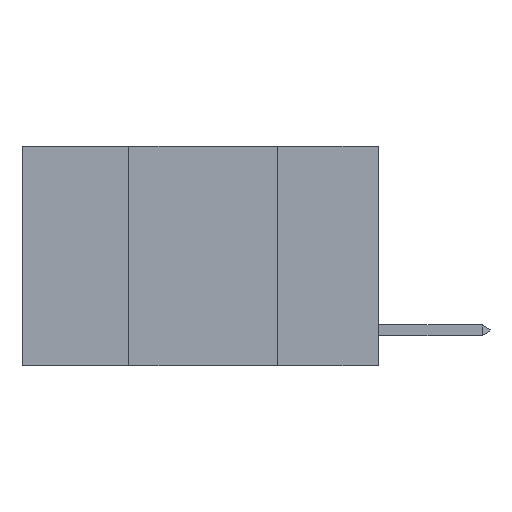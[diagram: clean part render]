
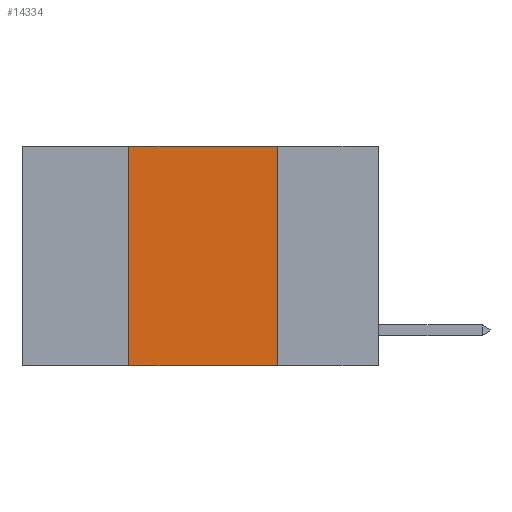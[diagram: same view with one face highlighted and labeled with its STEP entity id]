
A CAD part, left-side view. The second image highlights one B-rep face of the part: STEP entity #14334.
In plain terms, the highlighted planar face has unit normal (-1, 0, 0).
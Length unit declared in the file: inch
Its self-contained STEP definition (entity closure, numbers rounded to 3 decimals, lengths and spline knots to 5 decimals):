
#19 = DIRECTION ( 'NONE',  ( 0., 0., -1. ) ) ;
#130 = EDGE_LOOP ( 'NONE', ( #17119, #7793, #19392, #15109 ) ) ;
#524 = VECTOR ( 'NONE', #19965, 39.37008 ) ;
#1915 = VECTOR ( 'NONE', #15563, 39.37008 ) ;
#2830 = VERTEX_POINT ( 'NONE', #14378 ) ;
#3192 = DIRECTION ( 'NONE',  ( 0., -1., 0. ) ) ;
#3687 = PLANE ( 'NONE',  #16470 ) ;
#4139 = VERTEX_POINT ( 'NONE', #16263 ) ;
#4424 = LINE ( 'NONE', #21603, #18061 ) ;
#4474 = CARTESIAN_POINT ( 'NONE',  ( 0., 0.6, -0.37 ) ) ;
#5411 = LINE ( 'NONE', #4474, #15317 ) ;
#5548 = VERTEX_POINT ( 'NONE', #22966 ) ;
#6841 = LINE ( 'NONE', #8056, #1915 ) ;
#7793 = ORIENTED_EDGE ( 'NONE', *, *, #14755, .F. ) ;
#8056 = CARTESIAN_POINT ( 'NONE',  ( 0., 0.42, 0. ) ) ;
#8459 = VERTEX_POINT ( 'NONE', #21610 ) ;
#8909 = EDGE_CURVE ( 'NONE', #2830, #5548, #5411, .T. ) ;
#11141 = DIRECTION ( 'NONE',  ( 1., 0., 0. ) ) ;
#14334 = ADVANCED_FACE ( 'NONE', ( #22582 ), #3687, .F. ) ;
#14378 = CARTESIAN_POINT ( 'NONE',  ( 0., 0.42, -0.37 ) ) ;
#14755 = EDGE_CURVE ( 'NONE', #4139, #8459, #4424, .T. ) ;
#15109 = ORIENTED_EDGE ( 'NONE', *, *, #8909, .T. ) ;
#15317 = VECTOR ( 'NONE', #17469, 39.37008 ) ;
#15375 = LINE ( 'NONE', #18158, #524 ) ;
#15563 = DIRECTION ( 'NONE',  ( 0., 0., 1. ) ) ;
#16263 = CARTESIAN_POINT ( 'NONE',  ( 0., 0.42, 0. ) ) ;
#16401 = EDGE_CURVE ( 'NONE', #2830, #4139, #6841, .T. ) ;
#16470 = AXIS2_PLACEMENT_3D ( 'NONE', #16687, #11141, #19 ) ;
#16687 = CARTESIAN_POINT ( 'NONE',  ( 0., 0.6, 0. ) ) ;
#17119 = ORIENTED_EDGE ( 'NONE', *, *, #22796, .F. ) ;
#17469 = DIRECTION ( 'NONE',  ( 0., -1., 0. ) ) ;
#18061 = VECTOR ( 'NONE', #3192, 39.37008 ) ;
#18158 = CARTESIAN_POINT ( 'NONE',  ( 0., 0.17, 0. ) ) ;
#19392 = ORIENTED_EDGE ( 'NONE', *, *, #16401, .F. ) ;
#19965 = DIRECTION ( 'NONE',  ( 0., 0., -1. ) ) ;
#21603 = CARTESIAN_POINT ( 'NONE',  ( 0., 0.6, 0. ) ) ;
#21610 = CARTESIAN_POINT ( 'NONE',  ( 0., 0.17, 0. ) ) ;
#22582 = FACE_OUTER_BOUND ( 'NONE', #130, .T. ) ;
#22796 = EDGE_CURVE ( 'NONE', #8459, #5548, #15375, .T. ) ;
#22966 = CARTESIAN_POINT ( 'NONE',  ( 0., 0.17, -0.37 ) ) ;
